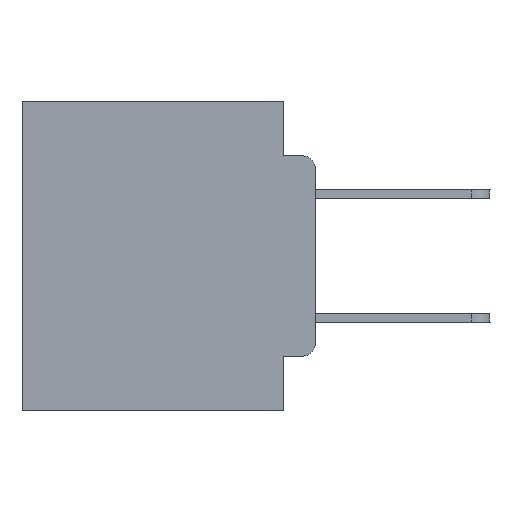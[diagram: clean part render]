
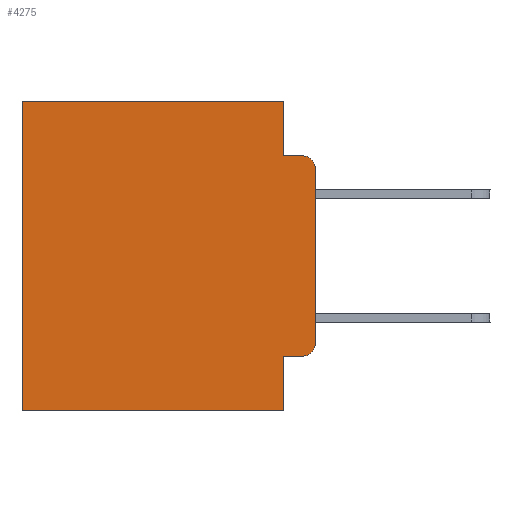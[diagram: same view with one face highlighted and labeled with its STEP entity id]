
A CAD part, left-side view. The second image highlights one B-rep face of the part: STEP entity #4275.
In plain terms, the highlighted planar face has unit normal (-1, 0, 0).
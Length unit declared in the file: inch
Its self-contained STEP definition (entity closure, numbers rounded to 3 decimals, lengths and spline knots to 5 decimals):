
#289 = CIRCLE ( 'NONE', #16025, 0.02 ) ;
#386 = VERTEX_POINT ( 'NONE', #15129 ) ;
#920 = ORIENTED_EDGE ( 'NONE', *, *, #15531, .T. ) ;
#969 = VECTOR ( 'NONE', #21001, 39.37008 ) ;
#2162 = DIRECTION ( 'NONE',  ( 0., -1., 0. ) ) ;
#2173 = VECTOR ( 'NONE', #14856, 39.37008 ) ;
#2613 = DIRECTION ( 'NONE',  ( 0., 0., -1. ) ) ;
#2667 = CIRCLE ( 'NONE', #4420, 0.02 ) ;
#3127 = EDGE_CURVE ( 'NONE', #386, #12381, #2667, .T. ) ;
#3136 = VERTEX_POINT ( 'NONE', #19894 ) ;
#3387 = VECTOR ( 'NONE', #24917, 39.37008 ) ;
#3434 = DIRECTION ( 'NONE',  ( 0., 0., -1. ) ) ;
#3519 = EDGE_CURVE ( 'NONE', #386, #3136, #13012, .T. ) ;
#3575 = CARTESIAN_POINT ( 'NONE',  ( 0.298, 0.02, -0.0885 ) ) ;
#4275 = ADVANCED_FACE ( 'NONE', ( #12505 ), #5245, .F. ) ;
#4392 = DIRECTION ( 'NONE',  ( 0., -1., 0. ) ) ;
#4420 = AXIS2_PLACEMENT_3D ( 'NONE', #11655, #26218, #3434 ) ;
#4583 = ORIENTED_EDGE ( 'NONE', *, *, #3519, .F. ) ;
#4694 = CARTESIAN_POINT ( 'NONE',  ( 0.298, 0., 0. ) ) ;
#4967 = DIRECTION ( 'NONE',  ( 1., 0., 0. ) ) ;
#5245 = PLANE ( 'NONE',  #5390 ) ;
#5390 = AXIS2_PLACEMENT_3D ( 'NONE', #4694, #4967, #25958 ) ;
#5445 = EDGE_CURVE ( 'NONE', #24025, #13445, #6625, .T. ) ;
#5451 = CARTESIAN_POINT ( 'NONE',  ( 0.298, 0.02, -0.3915 ) ) ;
#6625 = LINE ( 'NONE', #8947, #2173 ) ;
#6771 = LINE ( 'NONE', #19261, #21427 ) ;
#6993 = CARTESIAN_POINT ( 'NONE',  ( 0.298, 0.051, -0.5 ) ) ;
#7537 = ORIENTED_EDGE ( 'NONE', *, *, #8487, .F. ) ;
#8169 = LINE ( 'NONE', #16398, #3387 ) ;
#8289 = VECTOR ( 'NONE', #4392, 39.37008 ) ;
#8404 = CARTESIAN_POINT ( 'NONE',  ( 0.298, 0.051, 0. ) ) ;
#8477 = CARTESIAN_POINT ( 'NONE',  ( 0.298, 0.473, 0. ) ) ;
#8487 = EDGE_CURVE ( 'NONE', #12325, #21234, #6771, .T. ) ;
#8947 = CARTESIAN_POINT ( 'NONE',  ( 0.298, 0.473, 0. ) ) ;
#9522 = EDGE_CURVE ( 'NONE', #12131, #12381, #21508, .T. ) ;
#9642 = EDGE_CURVE ( 'NONE', #19353, #24025, #13686, .T. ) ;
#9675 = DIRECTION ( 'NONE',  ( 0., 0., -1. ) ) ;
#10699 = LINE ( 'NONE', #14961, #969 ) ;
#11476 = EDGE_LOOP ( 'NONE', ( #4583, #16789, #14793, #19617, #15300, #14446, #22463, #7537, #920, #25334 ) ) ;
#11655 = CARTESIAN_POINT ( 'NONE',  ( 0.298, 0.02, -0.1085 ) ) ;
#12131 = VERTEX_POINT ( 'NONE', #21017 ) ;
#12325 = VERTEX_POINT ( 'NONE', #13994 ) ;
#12381 = VERTEX_POINT ( 'NONE', #3575 ) ;
#12505 = FACE_OUTER_BOUND ( 'NONE', #11476, .T. ) ;
#13012 = LINE ( 'NONE', #21379, #25048 ) ;
#13081 = DIRECTION ( 'NONE',  ( 0., 0., -1. ) ) ;
#13319 = EDGE_CURVE ( 'NONE', #19353, #12131, #10699, .T. ) ;
#13445 = VERTEX_POINT ( 'NONE', #25264 ) ;
#13556 = CARTESIAN_POINT ( 'NONE',  ( 0.298, 0., 0. ) ) ;
#13686 = LINE ( 'NONE', #13556, #20849 ) ;
#13994 = CARTESIAN_POINT ( 'NONE',  ( 0.298, 0.051, -0.4115 ) ) ;
#14446 = ORIENTED_EDGE ( 'NONE', *, *, #5445, .T. ) ;
#14793 = ORIENTED_EDGE ( 'NONE', *, *, #9522, .F. ) ;
#14856 = DIRECTION ( 'NONE',  ( 0., 0., -1. ) ) ;
#14961 = CARTESIAN_POINT ( 'NONE',  ( 0.298, 0.051, 0. ) ) ;
#15129 = CARTESIAN_POINT ( 'NONE',  ( 0.298, 0., -0.1085 ) ) ;
#15213 = CARTESIAN_POINT ( 'NONE',  ( 0.298, 0.051, -0.0885 ) ) ;
#15300 = ORIENTED_EDGE ( 'NONE', *, *, #9642, .T. ) ;
#15531 = EDGE_CURVE ( 'NONE', #12325, #25220, #16557, .T. ) ;
#16025 = AXIS2_PLACEMENT_3D ( 'NONE', #5451, #22144, #9675 ) ;
#16398 = CARTESIAN_POINT ( 'NONE',  ( 0.298, 0., -0.5 ) ) ;
#16557 = LINE ( 'NONE', #24932, #25940 ) ;
#16789 = ORIENTED_EDGE ( 'NONE', *, *, #3127, .T. ) ;
#19261 = CARTESIAN_POINT ( 'NONE',  ( 0.298, 0.051, 0. ) ) ;
#19353 = VERTEX_POINT ( 'NONE', #8404 ) ;
#19617 = ORIENTED_EDGE ( 'NONE', *, *, #13319, .F. ) ;
#19739 = DIRECTION ( 'NONE',  ( 0., 1., 0. ) ) ;
#19894 = CARTESIAN_POINT ( 'NONE',  ( 0.298, 0., -0.3915 ) ) ;
#19984 = EDGE_CURVE ( 'NONE', #25220, #3136, #289, .T. ) ;
#20849 = VECTOR ( 'NONE', #19739, 39.37008 ) ;
#21001 = DIRECTION ( 'NONE',  ( 0., 0., -1. ) ) ;
#21017 = CARTESIAN_POINT ( 'NONE',  ( 0.298, 0.051, -0.0885 ) ) ;
#21234 = VERTEX_POINT ( 'NONE', #6993 ) ;
#21379 = CARTESIAN_POINT ( 'NONE',  ( 0.298, 0., 0. ) ) ;
#21427 = VECTOR ( 'NONE', #13081, 39.37008 ) ;
#21508 = LINE ( 'NONE', #15213, #8289 ) ;
#22144 = DIRECTION ( 'NONE',  ( -1., 0., 0. ) ) ;
#22463 = ORIENTED_EDGE ( 'NONE', *, *, #22542, .F. ) ;
#22542 = EDGE_CURVE ( 'NONE', #21234, #13445, #8169, .T. ) ;
#24025 = VERTEX_POINT ( 'NONE', #8477 ) ;
#24917 = DIRECTION ( 'NONE',  ( 0., 1., 0. ) ) ;
#24932 = CARTESIAN_POINT ( 'NONE',  ( 0.298, 0.051, -0.4115 ) ) ;
#25048 = VECTOR ( 'NONE', #2613, 39.37008 ) ;
#25220 = VERTEX_POINT ( 'NONE', #27017 ) ;
#25264 = CARTESIAN_POINT ( 'NONE',  ( 0.298, 0.473, -0.5 ) ) ;
#25334 = ORIENTED_EDGE ( 'NONE', *, *, #19984, .T. ) ;
#25940 = VECTOR ( 'NONE', #2162, 39.37008 ) ;
#25958 = DIRECTION ( 'NONE',  ( 0., 0., -1. ) ) ;
#26218 = DIRECTION ( 'NONE',  ( -1., 0., 0. ) ) ;
#27017 = CARTESIAN_POINT ( 'NONE',  ( 0.298, 0.02, -0.4115 ) ) ;
